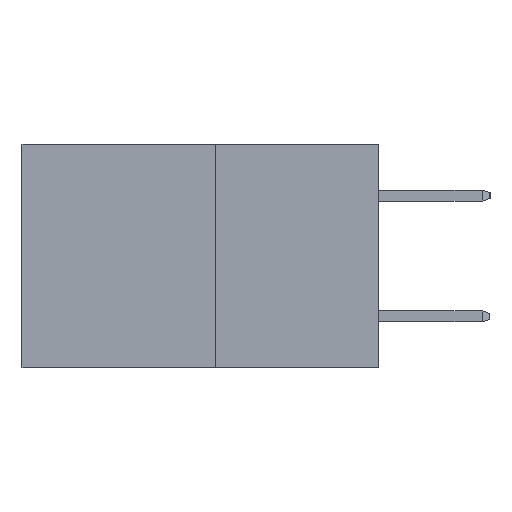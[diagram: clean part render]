
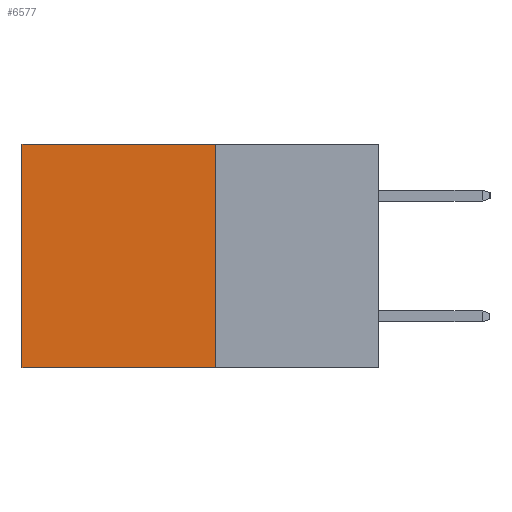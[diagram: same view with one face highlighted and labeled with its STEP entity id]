
A CAD part, left-side view. The second image highlights one B-rep face of the part: STEP entity #6577.
In plain terms, the highlighted planar face has unit normal (-1, 0, 0).
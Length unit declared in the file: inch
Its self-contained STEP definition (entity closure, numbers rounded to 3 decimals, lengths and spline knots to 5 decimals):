
#103 = LINE ( 'NONE', #5511, #10220 ) ;
#406 = VECTOR ( 'NONE', #8677, 39.37008 ) ;
#712 = LINE ( 'NONE', #9680, #406 ) ;
#1119 = LINE ( 'NONE', #10093, #11259 ) ;
#1355 = VERTEX_POINT ( 'NONE', #10588 ) ;
#1547 = FACE_OUTER_BOUND ( 'NONE', #12646, .T. ) ;
#2178 = EDGE_CURVE ( 'NONE', #3889, #7897, #103, .T. ) ;
#3889 = VERTEX_POINT ( 'NONE', #4390 ) ;
#4390 = CARTESIAN_POINT ( 'NONE',  ( 0.277, 0.27, 0. ) ) ;
#4626 = VECTOR ( 'NONE', #11220, 39.37008 ) ;
#4766 = CARTESIAN_POINT ( 'NONE',  ( 0.277, 0.27, -0.37 ) ) ;
#5022 = VERTEX_POINT ( 'NONE', #10532 ) ;
#5077 = EDGE_CURVE ( 'NONE', #7897, #1355, #1119, .T. ) ;
#5289 = ORIENTED_EDGE ( 'NONE', *, *, #2178, .F. ) ;
#5511 = CARTESIAN_POINT ( 'NONE',  ( 0.277, 0.27, -0.37 ) ) ;
#5530 = DIRECTION ( 'NONE',  ( 0., 0., -1. ) ) ;
#6288 = EDGE_CURVE ( 'NONE', #3889, #5022, #9806, .T. ) ;
#6577 = ADVANCED_FACE ( 'NONE', ( #1547 ), #7887, .F. ) ;
#6621 = ORIENTED_EDGE ( 'NONE', *, *, #5077, .F. ) ;
#7736 = DIRECTION ( 'NONE',  ( 0., 0., -1. ) ) ;
#7786 = DIRECTION ( 'NONE',  ( 1., 0., 0. ) ) ;
#7887 = PLANE ( 'NONE',  #8673 ) ;
#7897 = VERTEX_POINT ( 'NONE', #4766 ) ;
#7998 = CARTESIAN_POINT ( 'NONE',  ( 0.277, 0.27, -0.37 ) ) ;
#8661 = EDGE_CURVE ( 'NONE', #5022, #1355, #712, .T. ) ;
#8673 = AXIS2_PLACEMENT_3D ( 'NONE', #7998, #7786, #7736 ) ;
#8677 = DIRECTION ( 'NONE',  ( 0., 0., -1. ) ) ;
#9680 = CARTESIAN_POINT ( 'NONE',  ( 0.277, 0.59, -0.37 ) ) ;
#9806 = LINE ( 'NONE', #11447, #4626 ) ;
#10093 = CARTESIAN_POINT ( 'NONE',  ( 0.277, 0.27, -0.37 ) ) ;
#10106 = DIRECTION ( 'NONE',  ( 0., 1., 0. ) ) ;
#10220 = VECTOR ( 'NONE', #5530, 39.37008 ) ;
#10505 = ORIENTED_EDGE ( 'NONE', *, *, #6288, .T. ) ;
#10532 = CARTESIAN_POINT ( 'NONE',  ( 0.277, 0.59, 0. ) ) ;
#10588 = CARTESIAN_POINT ( 'NONE',  ( 0.277, 0.59, -0.37 ) ) ;
#11220 = DIRECTION ( 'NONE',  ( 0., 1., 0. ) ) ;
#11259 = VECTOR ( 'NONE', #10106, 39.37008 ) ;
#11447 = CARTESIAN_POINT ( 'NONE',  ( 0.277, 0.27, 0. ) ) ;
#11615 = ORIENTED_EDGE ( 'NONE', *, *, #8661, .T. ) ;
#12646 = EDGE_LOOP ( 'NONE', ( #11615, #6621, #5289, #10505 ) ) ;
